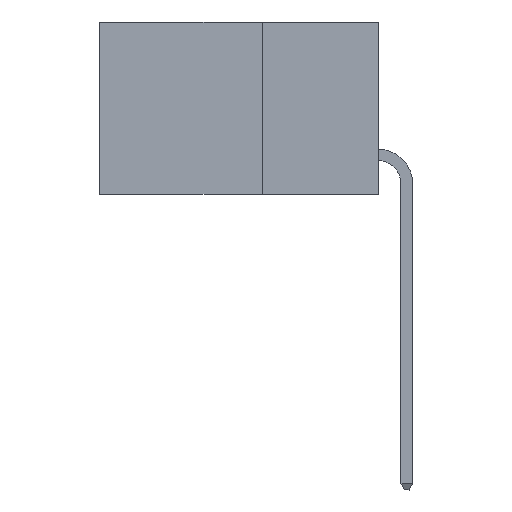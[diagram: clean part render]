
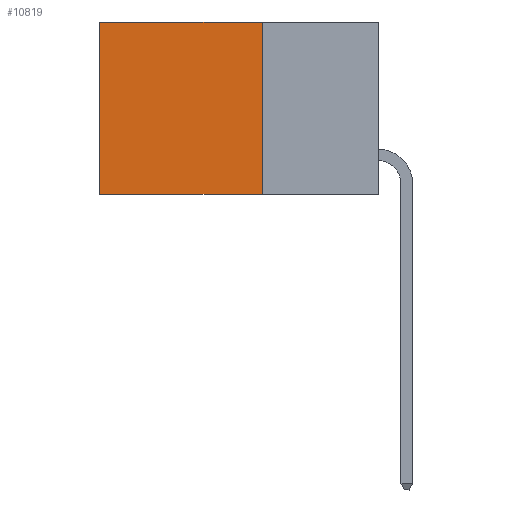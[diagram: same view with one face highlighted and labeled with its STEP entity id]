
A CAD part, left-side view. The second image highlights one B-rep face of the part: STEP entity #10819.
In plain terms, the highlighted planar face has unit normal (-1, 0, 0).
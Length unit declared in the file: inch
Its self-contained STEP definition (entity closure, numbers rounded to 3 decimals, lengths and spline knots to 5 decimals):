
#97 = ORIENTED_EDGE ( 'NONE', *, *, #1883, .T. ) ;
#394 = DIRECTION ( 'NONE',  ( 0., 1., 0. ) ) ;
#482 = VERTEX_POINT ( 'NONE', #6704 ) ;
#594 = CARTESIAN_POINT ( 'NONE',  ( 0.298, 0.25, 0. ) ) ;
#767 = EDGE_CURVE ( 'NONE', #482, #8669, #10591, .T. ) ;
#923 = AXIS2_PLACEMENT_3D ( 'NONE', #6996, #2290, #3208 ) ;
#1150 = DIRECTION ( 'NONE',  ( 0., 0., -1. ) ) ;
#1624 = CARTESIAN_POINT ( 'NONE',  ( 0.298, 0.6, -0.37 ) ) ;
#1883 = EDGE_CURVE ( 'NONE', #2700, #8669, #6271, .T. ) ;
#1887 = DIRECTION ( 'NONE',  ( 0., 0., -1. ) ) ;
#1895 = VECTOR ( 'NONE', #1887, 39.37008 ) ;
#2177 = VECTOR ( 'NONE', #11857, 39.37008 ) ;
#2290 = DIRECTION ( 'NONE',  ( 1., 0., 0. ) ) ;
#2700 = VERTEX_POINT ( 'NONE', #9251 ) ;
#2767 = ORIENTED_EDGE ( 'NONE', *, *, #767, .F. ) ;
#3014 = VECTOR ( 'NONE', #394, 39.37008 ) ;
#3208 = DIRECTION ( 'NONE',  ( 0., 0., -1. ) ) ;
#3588 = VECTOR ( 'NONE', #1150, 39.37008 ) ;
#3604 = EDGE_CURVE ( 'NONE', #10623, #482, #4413, .T. ) ;
#4247 = CARTESIAN_POINT ( 'NONE',  ( 0.298, 0.25, -0.37 ) ) ;
#4413 = LINE ( 'NONE', #9426, #1895 ) ;
#4919 = CARTESIAN_POINT ( 'NONE',  ( 0.298, 0.6, 0. ) ) ;
#5106 = PLANE ( 'NONE',  #923 ) ;
#5232 = CARTESIAN_POINT ( 'NONE',  ( 0.298, 0.25, 0. ) ) ;
#6271 = LINE ( 'NONE', #4919, #3588 ) ;
#6704 = CARTESIAN_POINT ( 'NONE',  ( 0.298, 0.25, -0.37 ) ) ;
#6850 = EDGE_LOOP ( 'NONE', ( #97, #2767, #9955, #9466 ) ) ;
#6996 = CARTESIAN_POINT ( 'NONE',  ( 0.298, 0.25, 0. ) ) ;
#7248 = LINE ( 'NONE', #5232, #2177 ) ;
#8669 = VERTEX_POINT ( 'NONE', #1624 ) ;
#9251 = CARTESIAN_POINT ( 'NONE',  ( 0.298, 0.6, 0. ) ) ;
#9426 = CARTESIAN_POINT ( 'NONE',  ( 0.298, 0.25, 0. ) ) ;
#9466 = ORIENTED_EDGE ( 'NONE', *, *, #12264, .T. ) ;
#9955 = ORIENTED_EDGE ( 'NONE', *, *, #3604, .F. ) ;
#10591 = LINE ( 'NONE', #4247, #3014 ) ;
#10623 = VERTEX_POINT ( 'NONE', #594 ) ;
#10698 = FACE_OUTER_BOUND ( 'NONE', #6850, .T. ) ;
#10819 = ADVANCED_FACE ( 'NONE', ( #10698 ), #5106, .F. ) ;
#11857 = DIRECTION ( 'NONE',  ( 0., 1., 0. ) ) ;
#12264 = EDGE_CURVE ( 'NONE', #10623, #2700, #7248, .T. ) ;
